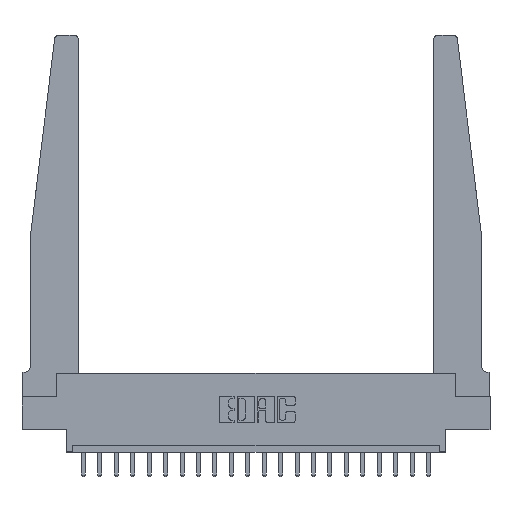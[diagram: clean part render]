
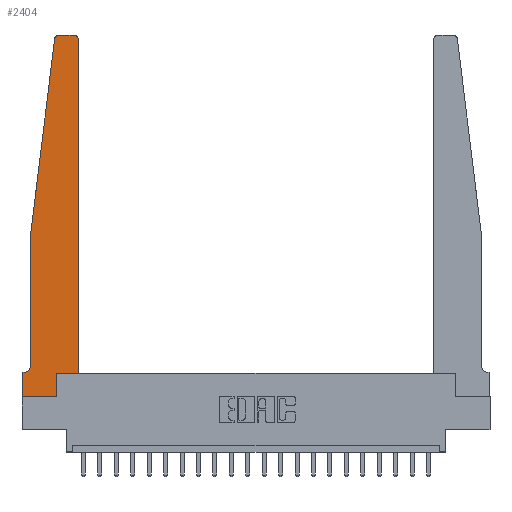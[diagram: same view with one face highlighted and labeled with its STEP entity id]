
A CAD part, top view. The second image highlights one B-rep face of the part: STEP entity #2404.
In plain terms, the highlighted planar face has unit normal (0, 0, 1).
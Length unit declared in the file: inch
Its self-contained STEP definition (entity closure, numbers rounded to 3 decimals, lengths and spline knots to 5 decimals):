
#296 = PLANE ( 'NONE',  #8118 ) ;
#544 = CARTESIAN_POINT ( 'NONE',  ( 0.2605, 0.18, 0.37 ) ) ;
#1119 = ORIENTED_EDGE ( 'NONE', *, *, #15054, .T. ) ;
#1362 = CARTESIAN_POINT ( 'NONE',  ( 0.25, 2.75, 0.37 ) ) ;
#1445 = AXIS2_PLACEMENT_3D ( 'NONE', #14557, #21306, #21517 ) ;
#1522 = DIRECTION ( 'NONE',  ( 0., 0., 1. ) ) ;
#1542 = DIRECTION ( 'NONE',  ( 1., 0., 0. ) ) ;
#1725 = DIRECTION ( 'NONE',  ( -0.122, -0.992, 0. ) ) ;
#1740 = EDGE_CURVE ( 'NONE', #10600, #15205, #20986, .T. ) ;
#1768 = ORIENTED_EDGE ( 'NONE', *, *, #16110, .T. ) ;
#1773 = DIRECTION ( 'NONE',  ( 1., 0., 0. ) ) ;
#1836 = VERTEX_POINT ( 'NONE', #17986 ) ;
#2091 = ORIENTED_EDGE ( 'NONE', *, *, #12947, .T. ) ;
#2099 = VERTEX_POINT ( 'NONE', #7268 ) ;
#2404 = ADVANCED_FACE ( 'NONE', ( #12157 ), #296, .T. ) ;
#2417 = LINE ( 'NONE', #544, #14759 ) ;
#2902 = DIRECTION ( 'NONE',  ( -1., 0., 0. ) ) ;
#3058 = CARTESIAN_POINT ( 'NONE',  ( 0.065, 1.25, 0.37 ) ) ;
#3159 = EDGE_CURVE ( 'NONE', #17010, #19477, #16347, .T. ) ;
#3643 = LINE ( 'NONE', #11953, #6979 ) ;
#4121 = VERTEX_POINT ( 'NONE', #4351 ) ;
#4177 = AXIS2_PLACEMENT_3D ( 'NONE', #8347, #1522, #4840 ) ;
#4229 = CARTESIAN_POINT ( 'NONE',  ( 0.065, 0.1875, 0.37 ) ) ;
#4351 = CARTESIAN_POINT ( 'NONE',  ( 0.2605, 0., 0.37 ) ) ;
#4526 = ORIENTED_EDGE ( 'NONE', *, *, #6336, .T. ) ;
#4699 = DIRECTION ( 'NONE',  ( 0., -1., 0. ) ) ;
#4840 = DIRECTION ( 'NONE',  ( 1., 0., 0. ) ) ;
#5330 = ORIENTED_EDGE ( 'NONE', *, *, #6788, .T. ) ;
#5963 = ORIENTED_EDGE ( 'NONE', *, *, #3159, .T. ) ;
#6099 = CARTESIAN_POINT ( 'NONE',  ( 0.2605, 0.18, 0.37 ) ) ;
#6240 = LINE ( 'NONE', #21660, #17359 ) ;
#6249 = EDGE_CURVE ( 'NONE', #19477, #14474, #10489, .T. ) ;
#6336 = EDGE_CURVE ( 'NONE', #11553, #17010, #20718, .T. ) ;
#6384 = DIRECTION ( 'NONE',  ( 0., 0., 1. ) ) ;
#6639 = VERTEX_POINT ( 'NONE', #11354 ) ;
#6754 = CARTESIAN_POINT ( 'NONE',  ( 0.425, 0.18, 0.37 ) ) ;
#6788 = EDGE_CURVE ( 'NONE', #6639, #11553, #15120, .T. ) ;
#6979 = VECTOR ( 'NONE', #1542, 39.37008 ) ;
#7268 = CARTESIAN_POINT ( 'NONE',  ( 0.065, 1.25, 0.37 ) ) ;
#7496 = DIRECTION ( 'NONE',  ( 0., 1., 0. ) ) ;
#7604 = CARTESIAN_POINT ( 'NONE',  ( 0.27653, 2.75, 0.37 ) ) ;
#7678 = CARTESIAN_POINT ( 'NONE',  ( 0.395, 2.75, 0.37 ) ) ;
#7749 = DIRECTION ( 'NONE',  ( -1., 0., 0. ) ) ;
#7902 = LINE ( 'NONE', #14613, #11224 ) ;
#8118 = AXIS2_PLACEMENT_3D ( 'NONE', #14051, #10532, #8994 ) ;
#8240 = LINE ( 'NONE', #3058, #8570 ) ;
#8347 = CARTESIAN_POINT ( 'NONE',  ( 0.27653, 2.72, 0.37 ) ) ;
#8419 = ORIENTED_EDGE ( 'NONE', *, *, #18776, .T. ) ;
#8570 = VECTOR ( 'NONE', #1725, 39.37008 ) ;
#8994 = DIRECTION ( 'NONE',  ( 1., 0., 0. ) ) ;
#9868 = EDGE_CURVE ( 'NONE', #20705, #6639, #16881, .T. ) ;
#10110 = CARTESIAN_POINT ( 'NONE',  ( 0.395, 2.72, 0.37 ) ) ;
#10235 = CARTESIAN_POINT ( 'NONE',  ( 0.425, 2.72, 0.37 ) ) ;
#10489 = CIRCLE ( 'NONE', #4177, 0.03 ) ;
#10532 = DIRECTION ( 'NONE',  ( 0., 0., 1. ) ) ;
#10600 = VERTEX_POINT ( 'NONE', #17719 ) ;
#10921 = CIRCLE ( 'NONE', #1445, 0.05 ) ;
#11224 = VECTOR ( 'NONE', #12836, 39.37008 ) ;
#11354 = CARTESIAN_POINT ( 'NONE',  ( 0.425, 0.18, 0.37 ) ) ;
#11507 = AXIS2_PLACEMENT_3D ( 'NONE', #10110, #6384, #13506 ) ;
#11519 = VECTOR ( 'NONE', #18976, 39.37008 ) ;
#11553 = VERTEX_POINT ( 'NONE', #10235 ) ;
#11953 = CARTESIAN_POINT ( 'NONE',  ( 0., 0., 0.37 ) ) ;
#12157 = FACE_OUTER_BOUND ( 'NONE', #15060, .T. ) ;
#12668 = VECTOR ( 'NONE', #2902, 39.37008 ) ;
#12836 = DIRECTION ( 'NONE',  ( 0., -1., 0. ) ) ;
#12947 = EDGE_CURVE ( 'NONE', #17580, #10600, #10921, .T. ) ;
#13506 = DIRECTION ( 'NONE',  ( 1., 0., 0. ) ) ;
#13536 = ORIENTED_EDGE ( 'NONE', *, *, #6249, .T. ) ;
#13546 = CARTESIAN_POINT ( 'NONE',  ( 0.24675, 2.72367, 0.37 ) ) ;
#14051 = CARTESIAN_POINT ( 'NONE',  ( 0., 0.1875, 0.37 ) ) ;
#14474 = VERTEX_POINT ( 'NONE', #13546 ) ;
#14557 = CARTESIAN_POINT ( 'NONE',  ( 0.015, 0.2375, 0.37 ) ) ;
#14613 = CARTESIAN_POINT ( 'NONE',  ( 0., 0., 0.37 ) ) ;
#14759 = VECTOR ( 'NONE', #7496, 39.37008 ) ;
#14986 = ORIENTED_EDGE ( 'NONE', *, *, #9868, .T. ) ;
#15054 = EDGE_CURVE ( 'NONE', #2099, #17580, #6240, .T. ) ;
#15060 = EDGE_LOOP ( 'NONE', ( #5963, #13536, #19958, #1119, #2091, #19835, #8419, #1768, #15692, #14986, #5330, #4526 ) ) ;
#15120 = LINE ( 'NONE', #6754, #11519 ) ;
#15205 = VERTEX_POINT ( 'NONE', #20666 ) ;
#15692 = ORIENTED_EDGE ( 'NONE', *, *, #18180, .T. ) ;
#15838 = VECTOR ( 'NONE', #7749, 39.37008 ) ;
#16110 = EDGE_CURVE ( 'NONE', #1836, #4121, #3643, .T. ) ;
#16347 = LINE ( 'NONE', #1362, #12668 ) ;
#16881 = LINE ( 'NONE', #20194, #17399 ) ;
#17010 = VERTEX_POINT ( 'NONE', #7678 ) ;
#17359 = VECTOR ( 'NONE', #4699, 39.37008 ) ;
#17399 = VECTOR ( 'NONE', #1773, 39.37008 ) ;
#17580 = VERTEX_POINT ( 'NONE', #20644 ) ;
#17719 = CARTESIAN_POINT ( 'NONE',  ( 0.015, 0.1875, 0.37 ) ) ;
#17986 = CARTESIAN_POINT ( 'NONE',  ( 0., 0., 0.37 ) ) ;
#18180 = EDGE_CURVE ( 'NONE', #4121, #20705, #2417, .T. ) ;
#18776 = EDGE_CURVE ( 'NONE', #15205, #1836, #7902, .T. ) ;
#18976 = DIRECTION ( 'NONE',  ( 0., 1., 0. ) ) ;
#19477 = VERTEX_POINT ( 'NONE', #7604 ) ;
#19835 = ORIENTED_EDGE ( 'NONE', *, *, #1740, .T. ) ;
#19958 = ORIENTED_EDGE ( 'NONE', *, *, #21207, .T. ) ;
#20194 = CARTESIAN_POINT ( 'NONE',  ( 0.425, 0.18, 0.37 ) ) ;
#20644 = CARTESIAN_POINT ( 'NONE',  ( 0.065, 0.2375, 0.37 ) ) ;
#20666 = CARTESIAN_POINT ( 'NONE',  ( 0., 0.1875, 0.37 ) ) ;
#20705 = VERTEX_POINT ( 'NONE', #6099 ) ;
#20718 = CIRCLE ( 'NONE', #11507, 0.03 ) ;
#20986 = LINE ( 'NONE', #4229, #15838 ) ;
#21207 = EDGE_CURVE ( 'NONE', #14474, #2099, #8240, .T. ) ;
#21306 = DIRECTION ( 'NONE',  ( 0., 0., -1. ) ) ;
#21517 = DIRECTION ( 'NONE',  ( -1., 0., 0. ) ) ;
#21660 = CARTESIAN_POINT ( 'NONE',  ( 0.065, 1.25, 0.37 ) ) ;
